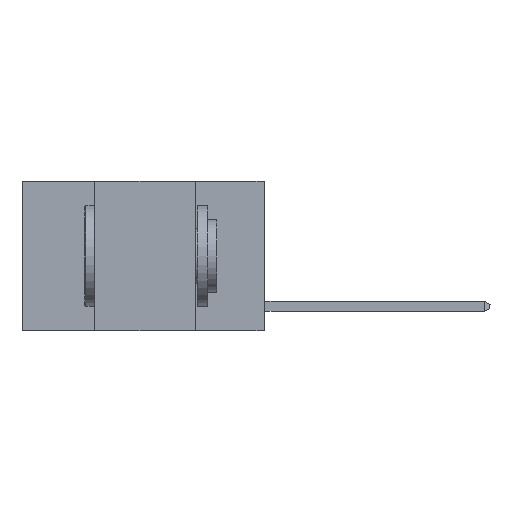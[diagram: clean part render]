
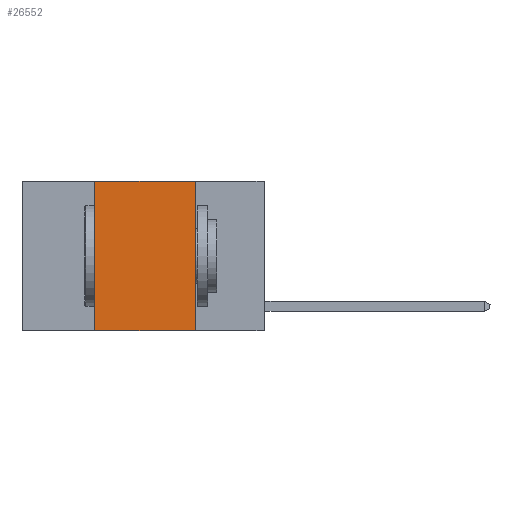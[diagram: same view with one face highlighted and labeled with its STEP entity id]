
A CAD part, left-side view. The second image highlights one B-rep face of the part: STEP entity #26552.
In plain terms, the highlighted planar face has unit normal (-1, 0, 0).
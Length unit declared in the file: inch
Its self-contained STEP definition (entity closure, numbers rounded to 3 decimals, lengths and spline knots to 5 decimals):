
#391 = LINE ( 'NONE', #2848, #18151 ) ;
#623 = EDGE_CURVE ( 'NONE', #26264, #15902, #9235, .T. ) ;
#2605 = DIRECTION ( 'NONE',  ( 0., 0., -1. ) ) ;
#2848 = CARTESIAN_POINT ( 'NONE',  ( 0., 0.6, 0. ) ) ;
#3375 = ORIENTED_EDGE ( 'NONE', *, *, #11166, .F. ) ;
#4196 = CARTESIAN_POINT ( 'NONE',  ( 0., 0.42, 0. ) ) ;
#4452 = EDGE_CURVE ( 'NONE', #9117, #15902, #18987, .T. ) ;
#4751 = ORIENTED_EDGE ( 'NONE', *, *, #5632, .F. ) ;
#4767 = FACE_OUTER_BOUND ( 'NONE', #4773, .T. ) ;
#4773 = EDGE_LOOP ( 'NONE', ( #26178, #4751, #3375, #28174 ) ) ;
#5632 = EDGE_CURVE ( 'NONE', #12229, #26264, #391, .T. ) ;
#7352 = CARTESIAN_POINT ( 'NONE',  ( 0., 0.42, 0. ) ) ;
#7615 = CARTESIAN_POINT ( 'NONE',  ( 0., 0.6, -0.37 ) ) ;
#7675 = AXIS2_PLACEMENT_3D ( 'NONE', #15993, #22545, #2605 ) ;
#9117 = VERTEX_POINT ( 'NONE', #25825 ) ;
#9235 = LINE ( 'NONE', #14037, #26280 ) ;
#11166 = EDGE_CURVE ( 'NONE', #9117, #12229, #14202, .T. ) ;
#12229 = VERTEX_POINT ( 'NONE', #4196 ) ;
#12366 = CARTESIAN_POINT ( 'NONE',  ( 0., 0.17, -0.37 ) ) ;
#12714 = VECTOR ( 'NONE', #23226, 39.37008 ) ;
#13637 = PLANE ( 'NONE',  #7675 ) ;
#14037 = CARTESIAN_POINT ( 'NONE',  ( 0., 0.17, 0. ) ) ;
#14202 = LINE ( 'NONE', #7352, #20893 ) ;
#15902 = VERTEX_POINT ( 'NONE', #12366 ) ;
#15993 = CARTESIAN_POINT ( 'NONE',  ( 0., 0.6, 0. ) ) ;
#16103 = DIRECTION ( 'NONE',  ( 0., -1., 0. ) ) ;
#16588 = CARTESIAN_POINT ( 'NONE',  ( 0., 0.17, 0. ) ) ;
#18151 = VECTOR ( 'NONE', #16103, 39.37008 ) ;
#18987 = LINE ( 'NONE', #7615, #12714 ) ;
#20601 = DIRECTION ( 'NONE',  ( 0., 0., -1. ) ) ;
#20893 = VECTOR ( 'NONE', #23100, 39.37008 ) ;
#22545 = DIRECTION ( 'NONE',  ( 1., 0., 0. ) ) ;
#23100 = DIRECTION ( 'NONE',  ( 0., 0., 1. ) ) ;
#23226 = DIRECTION ( 'NONE',  ( 0., -1., 0. ) ) ;
#25825 = CARTESIAN_POINT ( 'NONE',  ( 0., 0.42, -0.37 ) ) ;
#26178 = ORIENTED_EDGE ( 'NONE', *, *, #623, .F. ) ;
#26264 = VERTEX_POINT ( 'NONE', #16588 ) ;
#26280 = VECTOR ( 'NONE', #20601, 39.37008 ) ;
#26552 = ADVANCED_FACE ( 'NONE', ( #4767 ), #13637, .F. ) ;
#28174 = ORIENTED_EDGE ( 'NONE', *, *, #4452, .T. ) ;
